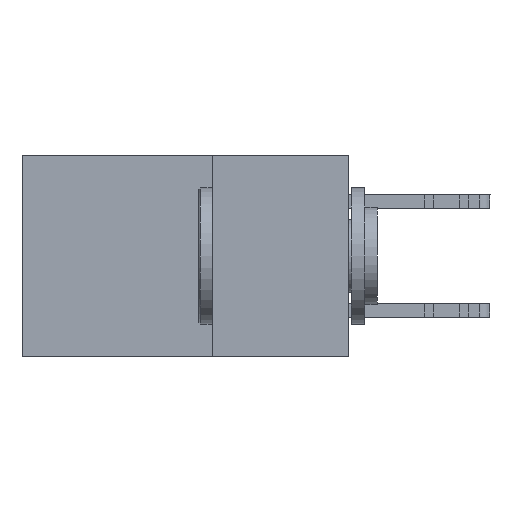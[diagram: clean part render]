
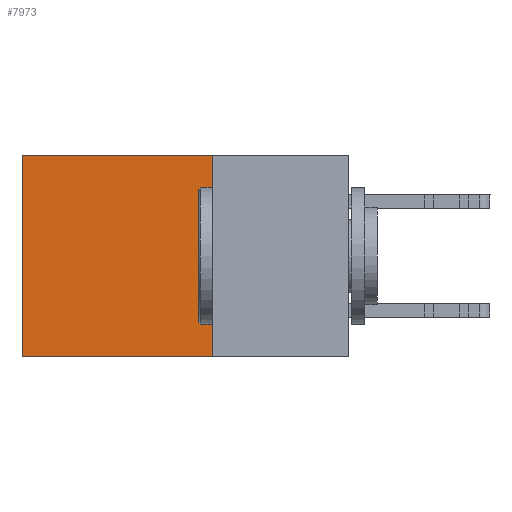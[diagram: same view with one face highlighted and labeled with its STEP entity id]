
A CAD part, left-side view. The second image highlights one B-rep face of the part: STEP entity #7973.
In plain terms, the highlighted planar face has unit normal (-1, 0, 0).
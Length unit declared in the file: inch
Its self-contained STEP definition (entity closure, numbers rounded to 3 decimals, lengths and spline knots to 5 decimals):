
#215 = DIRECTION ( 'NONE',  ( 0., 0., -1. ) ) ;
#967 = LINE ( 'NONE', #20411, #26766 ) ;
#3642 = DIRECTION ( 'NONE',  ( 0., 0., -1. ) ) ;
#6788 = VERTEX_POINT ( 'NONE', #26012 ) ;
#7973 = ADVANCED_FACE ( 'NONE', ( #21780 ), #21468, .F. ) ;
#8696 = ORIENTED_EDGE ( 'NONE', *, *, #27355, .F. ) ;
#9933 = DIRECTION ( 'NONE',  ( 0., 0., -1. ) ) ;
#12279 = DIRECTION ( 'NONE',  ( 1., 0., 0. ) ) ;
#14626 = CARTESIAN_POINT ( 'NONE',  ( 0.298, 0.25, 0. ) ) ;
#15045 = EDGE_CURVE ( 'NONE', #18099, #20776, #967, .T. ) ;
#15626 = CARTESIAN_POINT ( 'NONE',  ( 0.298, 0.6, -0.37 ) ) ;
#16388 = ORIENTED_EDGE ( 'NONE', *, *, #17987, .T. ) ;
#17967 = LINE ( 'NONE', #18276, #21834 ) ;
#17987 = EDGE_CURVE ( 'NONE', #28517, #6788, #17967, .T. ) ;
#18099 = VERTEX_POINT ( 'NONE', #18743 ) ;
#18276 = CARTESIAN_POINT ( 'NONE',  ( 0.298, 0.25, 0. ) ) ;
#18743 = CARTESIAN_POINT ( 'NONE',  ( 0.298, 0.25, -0.37 ) ) ;
#19314 = ORIENTED_EDGE ( 'NONE', *, *, #15045, .F. ) ;
#19502 = LINE ( 'NONE', #28686, #22889 ) ;
#20370 = VECTOR ( 'NONE', #3642, 39.37008 ) ;
#20411 = CARTESIAN_POINT ( 'NONE',  ( 0.298, 0.25, -0.37 ) ) ;
#20694 = ORIENTED_EDGE ( 'NONE', *, *, #26547, .T. ) ;
#20706 = LINE ( 'NONE', #25288, #20370 ) ;
#20776 = VERTEX_POINT ( 'NONE', #15626 ) ;
#21468 = PLANE ( 'NONE',  #23998 ) ;
#21780 = FACE_OUTER_BOUND ( 'NONE', #25341, .T. ) ;
#21834 = VECTOR ( 'NONE', #27897, 39.37008 ) ;
#22889 = VECTOR ( 'NONE', #215, 39.37008 ) ;
#23998 = AXIS2_PLACEMENT_3D ( 'NONE', #26619, #12279, #9933 ) ;
#25288 = CARTESIAN_POINT ( 'NONE',  ( 0.298, 0.25, 0. ) ) ;
#25341 = EDGE_LOOP ( 'NONE', ( #20694, #19314, #8696, #16388 ) ) ;
#25634 = DIRECTION ( 'NONE',  ( 0., 1., 0. ) ) ;
#26012 = CARTESIAN_POINT ( 'NONE',  ( 0.298, 0.6, 0. ) ) ;
#26547 = EDGE_CURVE ( 'NONE', #6788, #20776, #19502, .T. ) ;
#26619 = CARTESIAN_POINT ( 'NONE',  ( 0.298, 0.25, 0. ) ) ;
#26766 = VECTOR ( 'NONE', #25634, 39.37008 ) ;
#27355 = EDGE_CURVE ( 'NONE', #28517, #18099, #20706, .T. ) ;
#27897 = DIRECTION ( 'NONE',  ( 0., 1., 0. ) ) ;
#28517 = VERTEX_POINT ( 'NONE', #14626 ) ;
#28686 = CARTESIAN_POINT ( 'NONE',  ( 0.298, 0.6, 0. ) ) ;
